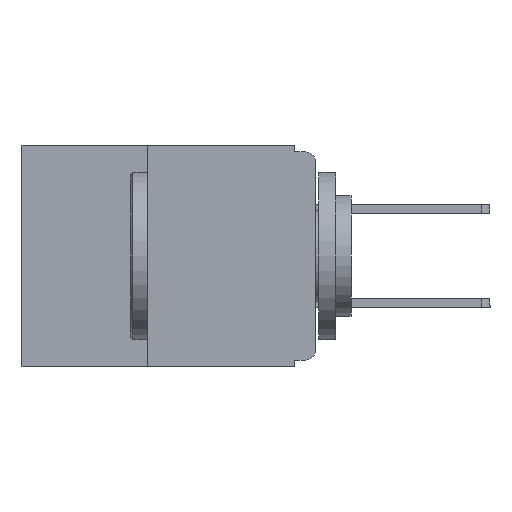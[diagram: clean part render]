
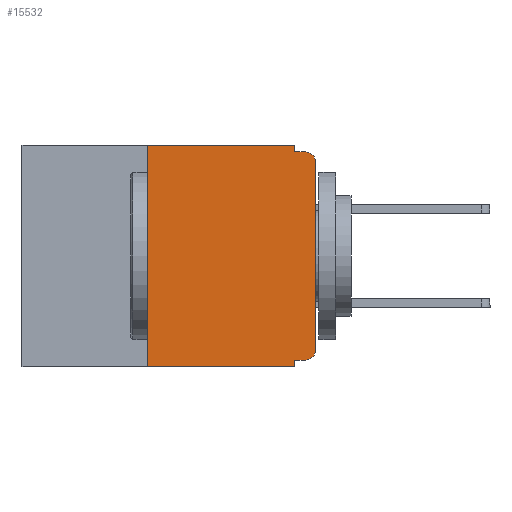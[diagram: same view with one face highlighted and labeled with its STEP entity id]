
A CAD part, left-side view. The second image highlights one B-rep face of the part: STEP entity #15532.
In plain terms, the highlighted planar face has unit normal (-1, 0, 0).
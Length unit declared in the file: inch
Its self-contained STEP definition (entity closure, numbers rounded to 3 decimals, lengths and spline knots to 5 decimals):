
#9 = VERTEX_POINT ( 'NONE', #25598 ) ;
#657 = CARTESIAN_POINT ( 'NONE',  ( 0., 0.031, 0. ) ) ;
#663 = DIRECTION ( 'NONE',  ( 0., 0., -1. ) ) ;
#710 = CARTESIAN_POINT ( 'NONE',  ( 0., 0.25, -0.33 ) ) ;
#2083 = AXIS2_PLACEMENT_3D ( 'NONE', #19965, #4824, #22525 ) ;
#2267 = VERTEX_POINT ( 'NONE', #31717 ) ;
#2960 = CARTESIAN_POINT ( 'NONE',  ( 0., 0., -0.01 ) ) ;
#2984 = AXIS2_PLACEMENT_3D ( 'NONE', #11213, #31317, #16355 ) ;
#3491 = LINE ( 'NONE', #31311, #9372 ) ;
#3799 = EDGE_CURVE ( 'NONE', #24419, #2267, #11264, .T. ) ;
#4584 = VECTOR ( 'NONE', #10718, 39.37008 ) ;
#4611 = EDGE_CURVE ( 'NONE', #26623, #9024, #27825, .T. ) ;
#4682 = CARTESIAN_POINT ( 'NONE',  ( 0., 0.25, -0.33 ) ) ;
#4824 = DIRECTION ( 'NONE',  ( -1., 0., 0. ) ) ;
#5484 = DIRECTION ( 'NONE',  ( 0., -1., 0. ) ) ;
#5646 = FACE_OUTER_BOUND ( 'NONE', #24301, .T. ) ;
#6330 = ORIENTED_EDGE ( 'NONE', *, *, #15759, .T. ) ;
#7091 = ORIENTED_EDGE ( 'NONE', *, *, #4611, .T. ) ;
#7176 = DIRECTION ( 'NONE',  ( 0., 0., 1. ) ) ;
#8116 = VERTEX_POINT ( 'NONE', #8963 ) ;
#8193 = CIRCLE ( 'NONE', #2083, 0.015 ) ;
#8437 = CARTESIAN_POINT ( 'NONE',  ( 0., 0.031, -0.01 ) ) ;
#8963 = CARTESIAN_POINT ( 'NONE',  ( 0., 0.015, -0.01 ) ) ;
#9024 = VERTEX_POINT ( 'NONE', #21146 ) ;
#9160 = CARTESIAN_POINT ( 'NONE',  ( 0., 0.437, 0. ) ) ;
#9372 = VECTOR ( 'NONE', #11207, 39.37008 ) ;
#9690 = VECTOR ( 'NONE', #26890, 39.37008 ) ;
#10060 = VECTOR ( 'NONE', #16656, 39.37008 ) ;
#10084 = CARTESIAN_POINT ( 'NONE',  ( 0., 0.015, -0.305 ) ) ;
#10459 = VECTOR ( 'NONE', #7176, 39.37008 ) ;
#10718 = DIRECTION ( 'NONE',  ( 0., 0., -1. ) ) ;
#11207 = DIRECTION ( 'NONE',  ( 0., -1., 0. ) ) ;
#11213 = CARTESIAN_POINT ( 'NONE',  ( 0., 0.437, 0. ) ) ;
#11264 = LINE ( 'NONE', #30753, #4584 ) ;
#11310 = ORIENTED_EDGE ( 'NONE', *, *, #14450, .F. ) ;
#11637 = EDGE_CURVE ( 'NONE', #20595, #15994, #13332, .T. ) ;
#11747 = EDGE_CURVE ( 'NONE', #19193, #2267, #3491, .T. ) ;
#12020 = EDGE_CURVE ( 'NONE', #9024, #8116, #8193, .T. ) ;
#12613 = DIRECTION ( 'NONE',  ( 0., 0., -1. ) ) ;
#13332 = LINE ( 'NONE', #657, #26845 ) ;
#13730 = PLANE ( 'NONE',  #2984 ) ;
#14026 = ORIENTED_EDGE ( 'NONE', *, *, #15342, .F. ) ;
#14236 = EDGE_CURVE ( 'NONE', #29715, #24419, #16867, .T. ) ;
#14309 = CIRCLE ( 'NONE', #30014, 0.015 ) ;
#14450 = EDGE_CURVE ( 'NONE', #19193, #9, #30549, .T. ) ;
#14629 = CARTESIAN_POINT ( 'NONE',  ( 0., 0.031, -0.32 ) ) ;
#15342 = EDGE_CURVE ( 'NONE', #15994, #8116, #23901, .T. ) ;
#15532 = ADVANCED_FACE ( 'NONE', ( #5646 ), #13730, .F. ) ;
#15759 = EDGE_CURVE ( 'NONE', #29715, #26623, #14309, .T. ) ;
#15994 = VERTEX_POINT ( 'NONE', #8437 ) ;
#16355 = DIRECTION ( 'NONE',  ( 0., 0., -1. ) ) ;
#16656 = DIRECTION ( 'NONE',  ( 0., 1., 0. ) ) ;
#16867 = LINE ( 'NONE', #26676, #10060 ) ;
#17175 = VECTOR ( 'NONE', #5484, 39.37008 ) ;
#17503 = EDGE_CURVE ( 'NONE', #9, #20595, #29064, .T. ) ;
#19193 = VERTEX_POINT ( 'NONE', #710 ) ;
#19610 = ORIENTED_EDGE ( 'NONE', *, *, #11637, .F. ) ;
#19965 = CARTESIAN_POINT ( 'NONE',  ( 0., 0.015, -0.025 ) ) ;
#20371 = VECTOR ( 'NONE', #30671, 39.37008 ) ;
#20521 = CARTESIAN_POINT ( 'NONE',  ( 0., 0.031, 0. ) ) ;
#20595 = VERTEX_POINT ( 'NONE', #20521 ) ;
#20730 = ORIENTED_EDGE ( 'NONE', *, *, #14236, .F. ) ;
#21146 = CARTESIAN_POINT ( 'NONE',  ( 0., 0., -0.025 ) ) ;
#22144 = ORIENTED_EDGE ( 'NONE', *, *, #11747, .T. ) ;
#22525 = DIRECTION ( 'NONE',  ( 0., 0., -1. ) ) ;
#23901 = LINE ( 'NONE', #2960, #17175 ) ;
#24301 = EDGE_LOOP ( 'NONE', ( #7091, #31460, #14026, #19610, #24659, #11310, #22144, #30952, #20730, #6330 ) ) ;
#24419 = VERTEX_POINT ( 'NONE', #14629 ) ;
#24659 = ORIENTED_EDGE ( 'NONE', *, *, #17503, .F. ) ;
#25598 = CARTESIAN_POINT ( 'NONE',  ( 0., 0.25, 0. ) ) ;
#26623 = VERTEX_POINT ( 'NONE', #31583 ) ;
#26676 = CARTESIAN_POINT ( 'NONE',  ( 0., 0., -0.32 ) ) ;
#26845 = VECTOR ( 'NONE', #663, 39.37008 ) ;
#26890 = DIRECTION ( 'NONE',  ( 0., -1., 0. ) ) ;
#27787 = DIRECTION ( 'NONE',  ( -1., 0., 0. ) ) ;
#27825 = LINE ( 'NONE', #31400, #20371 ) ;
#29064 = LINE ( 'NONE', #9160, #9690 ) ;
#29715 = VERTEX_POINT ( 'NONE', #32354 ) ;
#30014 = AXIS2_PLACEMENT_3D ( 'NONE', #10084, #27787, #12613 ) ;
#30549 = LINE ( 'NONE', #4682, #10459 ) ;
#30671 = DIRECTION ( 'NONE',  ( 0., 0., 1. ) ) ;
#30753 = CARTESIAN_POINT ( 'NONE',  ( 0., 0.031, -0.33 ) ) ;
#30952 = ORIENTED_EDGE ( 'NONE', *, *, #3799, .F. ) ;
#31311 = CARTESIAN_POINT ( 'NONE',  ( 0., 0.437, -0.33 ) ) ;
#31317 = DIRECTION ( 'NONE',  ( 1., 0., 0. ) ) ;
#31400 = CARTESIAN_POINT ( 'NONE',  ( 0., 0., 0. ) ) ;
#31460 = ORIENTED_EDGE ( 'NONE', *, *, #12020, .T. ) ;
#31583 = CARTESIAN_POINT ( 'NONE',  ( 0., 0., -0.305 ) ) ;
#31717 = CARTESIAN_POINT ( 'NONE',  ( 0., 0.031, -0.33 ) ) ;
#32354 = CARTESIAN_POINT ( 'NONE',  ( 0., 0.015, -0.32 ) ) ;
